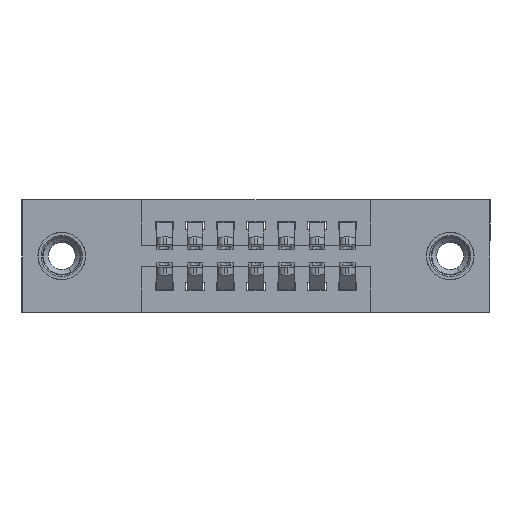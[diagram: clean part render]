
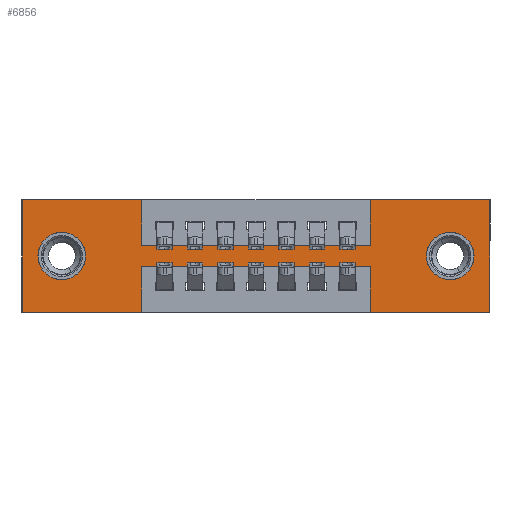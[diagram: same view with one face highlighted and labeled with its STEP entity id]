
A CAD part, front view. The second image highlights one B-rep face of the part: STEP entity #6856.
In plain terms, the highlighted planar face has unit normal (0, -1, 0).
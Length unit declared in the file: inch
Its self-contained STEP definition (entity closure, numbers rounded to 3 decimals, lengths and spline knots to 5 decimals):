
#71 = VERTEX_POINT ( 'NONE', #7744 ) ;
#281 = VERTEX_POINT ( 'NONE', #8803 ) ;
#354 = LINE ( 'NONE', #2320, #10541 ) ;
#412 = CARTESIAN_POINT ( 'NONE',  ( 0.3925, 0., -0.15 ) ) ;
#526 = CARTESIAN_POINT ( 'NONE',  ( 0.3925, 0., -0.22 ) ) ;
#553 = DIRECTION ( 'NONE',  ( 0., 0., 1. ) ) ;
#614 = DIRECTION ( 'NONE',  ( 0., 0., -1. ) ) ;
#667 = LINE ( 'NONE', #8917, #10801 ) ;
#939 = VERTEX_POINT ( 'NONE', #2914 ) ;
#981 = DIRECTION ( 'NONE',  ( 0., 1., 0. ) ) ;
#1081 = ORIENTED_EDGE ( 'NONE', *, *, #8703, .F. ) ;
#1183 = LINE ( 'NONE', #4127, #11251 ) ;
#1212 = CARTESIAN_POINT ( 'NONE',  ( 0.3925, 0., -0.15 ) ) ;
#1233 = CARTESIAN_POINT ( 'NONE',  ( 0.13, 0., -0.107 ) ) ;
#1292 = LINE ( 'NONE', #5829, #4009 ) ;
#1376 = EDGE_CURVE ( 'NONE', #7895, #6576, #1183, .T. ) ;
#1432 = ORIENTED_EDGE ( 'NONE', *, *, #3490, .T. ) ;
#1451 = DIRECTION ( 'NONE',  ( 1., 0., 0. ) ) ;
#1506 = CARTESIAN_POINT ( 'NONE',  ( 0., 0., 0. ) ) ;
#1657 = CARTESIAN_POINT ( 'NONE',  ( 0.3925, 0., 0. ) ) ;
#1859 = VECTOR ( 'NONE', #1451, 39.37008 ) ;
#1928 = LINE ( 'NONE', #10514, #12229 ) ;
#2103 = ORIENTED_EDGE ( 'NONE', *, *, #9281, .F. ) ;
#2171 = VECTOR ( 'NONE', #3604, 39.37008 ) ;
#2320 = CARTESIAN_POINT ( 'NONE',  ( 0., 0., 0. ) ) ;
#2481 = EDGE_CURVE ( 'NONE', #4581, #3482, #6860, .T. ) ;
#2544 = CARTESIAN_POINT ( 'NONE',  ( 0., 0., 0. ) ) ;
#2582 = ORIENTED_EDGE ( 'NONE', *, *, #2481, .F. ) ;
#2588 = ORIENTED_EDGE ( 'NONE', *, *, #7131, .T. ) ;
#2738 = CIRCLE ( 'NONE', #11284, 0.078 ) ;
#2780 = VECTOR ( 'NONE', #4525, 39.37008 ) ;
#2914 = CARTESIAN_POINT ( 'NONE',  ( 0.13, 0., -0.263 ) ) ;
#2917 = EDGE_CURVE ( 'NONE', #71, #12281, #7149, .T. ) ;
#2944 = VERTEX_POINT ( 'NONE', #1233 ) ;
#3038 = ORIENTED_EDGE ( 'NONE', *, *, #1376, .F. ) ;
#3297 = CARTESIAN_POINT ( 'NONE',  ( 1.1425, 0., -0.15 ) ) ;
#3357 = ORIENTED_EDGE ( 'NONE', *, *, #5151, .F. ) ;
#3476 = CARTESIAN_POINT ( 'NONE',  ( 0., 0., -0.37 ) ) ;
#3482 = VERTEX_POINT ( 'NONE', #6075 ) ;
#3490 = EDGE_CURVE ( 'NONE', #5653, #9038, #3600, .T. ) ;
#3600 = CIRCLE ( 'NONE', #4553, 0.078 ) ;
#3604 = DIRECTION ( 'NONE',  ( 0., 0., 1. ) ) ;
#3741 = CARTESIAN_POINT ( 'NONE',  ( 1.1425, 0., -0.37 ) ) ;
#3802 = VERTEX_POINT ( 'NONE', #1212 ) ;
#3853 = FACE_OUTER_BOUND ( 'NONE', #12432, .T. ) ;
#3893 = ORIENTED_EDGE ( 'NONE', *, *, #10608, .F. ) ;
#3949 = CARTESIAN_POINT ( 'NONE',  ( 0.13, 0., -0.185 ) ) ;
#4009 = VECTOR ( 'NONE', #6795, 39.37008 ) ;
#4048 = DIRECTION ( 'NONE',  ( -1., 0., 0. ) ) ;
#4127 = CARTESIAN_POINT ( 'NONE',  ( 0., 0., -0.37 ) ) ;
#4140 = DIRECTION ( 'NONE',  ( 0., 1., 0. ) ) ;
#4243 = LINE ( 'NONE', #2544, #2171 ) ;
#4256 = VECTOR ( 'NONE', #8506, 39.37008 ) ;
#4389 = VECTOR ( 'NONE', #553, 39.37008 ) ;
#4525 = DIRECTION ( 'NONE',  ( 1., 0., 0. ) ) ;
#4553 = AXIS2_PLACEMENT_3D ( 'NONE', #7811, #7797, #7769 ) ;
#4581 = VERTEX_POINT ( 'NONE', #526 ) ;
#4645 = CARTESIAN_POINT ( 'NONE',  ( 1.1425, 0., -0.37 ) ) ;
#4658 = VECTOR ( 'NONE', #10090, 39.37008 ) ;
#4951 = DIRECTION ( 'NONE',  ( 0., 0., 1. ) ) ;
#4965 = LINE ( 'NONE', #11979, #4658 ) ;
#5094 = DIRECTION ( 'NONE',  ( 0., 0., 1. ) ) ;
#5151 = EDGE_CURVE ( 'NONE', #3802, #6735, #10199, .T. ) ;
#5253 = CARTESIAN_POINT ( 'NONE',  ( 1.405, 0., -0.107 ) ) ;
#5405 = AXIS2_PLACEMENT_3D ( 'NONE', #9904, #4140, #10836 ) ;
#5487 = DIRECTION ( 'NONE',  ( 0., -1., 0. ) ) ;
#5653 = VERTEX_POINT ( 'NONE', #10980 ) ;
#5713 = CIRCLE ( 'NONE', #8133, 0.078 ) ;
#5829 = CARTESIAN_POINT ( 'NONE',  ( 0., 0., -0.37 ) ) ;
#6075 = CARTESIAN_POINT ( 'NONE',  ( 0.3925, 0., -0.37 ) ) ;
#6241 = ORIENTED_EDGE ( 'NONE', *, *, #9840, .F. ) ;
#6342 = DIRECTION ( 'NONE',  ( 1., 0., 0. ) ) ;
#6471 = AXIS2_PLACEMENT_3D ( 'NONE', #3476, #5487, #12105 ) ;
#6576 = VERTEX_POINT ( 'NONE', #3741 ) ;
#6632 = EDGE_CURVE ( 'NONE', #3482, #12461, #1292, .T. ) ;
#6651 = EDGE_CURVE ( 'NONE', #9038, #5653, #11643, .T. ) ;
#6735 = VERTEX_POINT ( 'NONE', #3297 ) ;
#6795 = DIRECTION ( 'NONE',  ( -1., 0., 0. ) ) ;
#6856 = ADVANCED_FACE ( 'NONE', ( #11191, #11494, #3853 ), #11158, .T. ) ;
#6860 = LINE ( 'NONE', #8527, #4256 ) ;
#7000 = CARTESIAN_POINT ( 'NONE',  ( 0.13, 0., -0.185 ) ) ;
#7081 = CARTESIAN_POINT ( 'NONE',  ( 0., 0., -0.37 ) ) ;
#7131 = EDGE_CURVE ( 'NONE', #939, #2944, #5713, .T. ) ;
#7149 = LINE ( 'NONE', #1506, #1859 ) ;
#7189 = EDGE_CURVE ( 'NONE', #2944, #939, #2738, .T. ) ;
#7211 = ORIENTED_EDGE ( 'NONE', *, *, #6632, .F. ) ;
#7225 = CARTESIAN_POINT ( 'NONE',  ( 1.535, 0., -0.37 ) ) ;
#7744 = CARTESIAN_POINT ( 'NONE',  ( 1.1425, 0., 0. ) ) ;
#7769 = DIRECTION ( 'NONE',  ( 0., 0., -1. ) ) ;
#7797 = DIRECTION ( 'NONE',  ( 0., 1., 0. ) ) ;
#7811 = CARTESIAN_POINT ( 'NONE',  ( 1.405, 0., -0.185 ) ) ;
#7895 = VERTEX_POINT ( 'NONE', #7225 ) ;
#7940 = DIRECTION ( 'NONE',  ( 0., 0., 1. ) ) ;
#8052 = ORIENTED_EDGE ( 'NONE', *, *, #2917, .F. ) ;
#8133 = AXIS2_PLACEMENT_3D ( 'NONE', #3949, #10662, #4951 ) ;
#8506 = DIRECTION ( 'NONE',  ( 0., 0., -1. ) ) ;
#8527 = CARTESIAN_POINT ( 'NONE',  ( 0.3925, 0., -0.37 ) ) ;
#8554 = EDGE_CURVE ( 'NONE', #10291, #281, #354, .T. ) ;
#8602 = CARTESIAN_POINT ( 'NONE',  ( 1.1425, 0., -0.22 ) ) ;
#8703 = EDGE_CURVE ( 'NONE', #12461, #10291, #4243, .T. ) ;
#8803 = CARTESIAN_POINT ( 'NONE',  ( 0.3925, 0., 0. ) ) ;
#8917 = CARTESIAN_POINT ( 'NONE',  ( 1.1425, 0., 0. ) ) ;
#8959 = ORIENTED_EDGE ( 'NONE', *, *, #8554, .F. ) ;
#9038 = VERTEX_POINT ( 'NONE', #5253 ) ;
#9281 = EDGE_CURVE ( 'NONE', #6576, #10857, #9488, .T. ) ;
#9488 = LINE ( 'NONE', #4645, #4389 ) ;
#9550 = ORIENTED_EDGE ( 'NONE', *, *, #6651, .T. ) ;
#9567 = EDGE_LOOP ( 'NONE', ( #9550, #1432 ) ) ;
#9609 = CARTESIAN_POINT ( 'NONE',  ( 0., 0., 0. ) ) ;
#9840 = EDGE_CURVE ( 'NONE', #6735, #71, #667, .T. ) ;
#9883 = EDGE_LOOP ( 'NONE', ( #10603, #2588 ) ) ;
#9904 = CARTESIAN_POINT ( 'NONE',  ( 1.405, 0., -0.185 ) ) ;
#10090 = DIRECTION ( 'NONE',  ( -1., 0., 0. ) ) ;
#10199 = LINE ( 'NONE', #412, #2780 ) ;
#10209 = EDGE_CURVE ( 'NONE', #281, #3802, #12264, .T. ) ;
#10291 = VERTEX_POINT ( 'NONE', #9609 ) ;
#10514 = CARTESIAN_POINT ( 'NONE',  ( 1.535, 0., 0. ) ) ;
#10541 = VECTOR ( 'NONE', #6342, 39.37008 ) ;
#10603 = ORIENTED_EDGE ( 'NONE', *, *, #7189, .T. ) ;
#10608 = EDGE_CURVE ( 'NONE', #10857, #4581, #4965, .T. ) ;
#10662 = DIRECTION ( 'NONE',  ( 0., 1., 0. ) ) ;
#10713 = ORIENTED_EDGE ( 'NONE', *, *, #10209, .F. ) ;
#10747 = CARTESIAN_POINT ( 'NONE',  ( 1.535, 0., 0. ) ) ;
#10801 = VECTOR ( 'NONE', #5094, 39.37008 ) ;
#10836 = DIRECTION ( 'NONE',  ( 0., 0., -1. ) ) ;
#10857 = VERTEX_POINT ( 'NONE', #8602 ) ;
#10980 = CARTESIAN_POINT ( 'NONE',  ( 1.405, 0., -0.263 ) ) ;
#11158 = PLANE ( 'NONE',  #6471 ) ;
#11191 = FACE_BOUND ( 'NONE', #9567, .T. ) ;
#11251 = VECTOR ( 'NONE', #4048, 39.37008 ) ;
#11284 = AXIS2_PLACEMENT_3D ( 'NONE', #7000, #981, #7940 ) ;
#11494 = FACE_BOUND ( 'NONE', #9883, .T. ) ;
#11546 = EDGE_CURVE ( 'NONE', #12281, #7895, #1928, .T. ) ;
#11643 = CIRCLE ( 'NONE', #5405, 0.078 ) ;
#11974 = VECTOR ( 'NONE', #614, 39.37008 ) ;
#11979 = CARTESIAN_POINT ( 'NONE',  ( 0.3925, 0., -0.22 ) ) ;
#12105 = DIRECTION ( 'NONE',  ( 0., 0., -1. ) ) ;
#12229 = VECTOR ( 'NONE', #12359, 39.37008 ) ;
#12264 = LINE ( 'NONE', #1657, #11974 ) ;
#12281 = VERTEX_POINT ( 'NONE', #10747 ) ;
#12289 = ORIENTED_EDGE ( 'NONE', *, *, #11546, .F. ) ;
#12359 = DIRECTION ( 'NONE',  ( 0., 0., -1. ) ) ;
#12432 = EDGE_LOOP ( 'NONE', ( #2582, #3893, #2103, #3038, #12289, #8052, #6241, #3357, #10713, #8959, #1081, #7211 ) ) ;
#12461 = VERTEX_POINT ( 'NONE', #7081 ) ;
